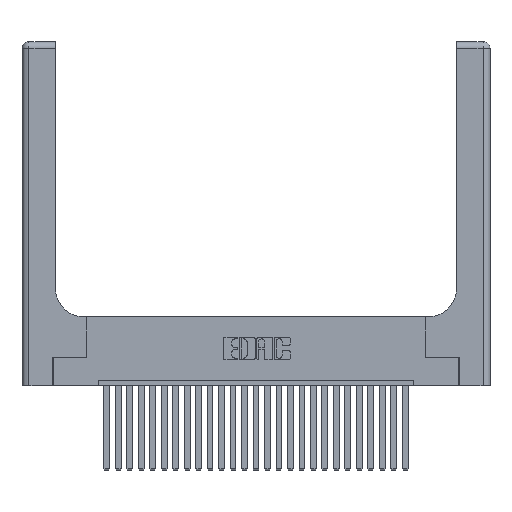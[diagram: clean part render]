
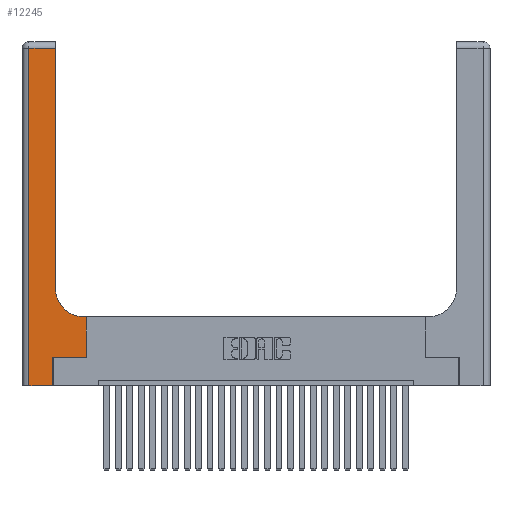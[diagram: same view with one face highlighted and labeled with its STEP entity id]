
A CAD part, top view. The second image highlights one B-rep face of the part: STEP entity #12245.
In plain terms, the highlighted planar face has unit normal (0, 0, 1).
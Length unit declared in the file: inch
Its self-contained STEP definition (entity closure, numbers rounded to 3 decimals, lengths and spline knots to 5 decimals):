
#540 = CARTESIAN_POINT ( 'NONE',  ( 0., 2.94, 0.37 ) ) ;
#699 = LINE ( 'NONE', #5644, #4050 ) ;
#837 = DIRECTION ( 'NONE',  ( 1., 0., 0. ) ) ;
#869 = PLANE ( 'NONE',  #12640 ) ;
#1617 = LINE ( 'NONE', #21561, #12179 ) ;
#1692 = VERTEX_POINT ( 'NONE', #2813 ) ;
#1924 = EDGE_CURVE ( 'NONE', #6714, #13691, #11876, .T. ) ;
#2122 = ORIENTED_EDGE ( 'NONE', *, *, #11858, .T. ) ;
#2713 = CARTESIAN_POINT ( 'NONE',  ( 0.5415, 0.85, 0.37 ) ) ;
#2813 = CARTESIAN_POINT ( 'NONE',  ( 0.5415, 0.6, 0.37 ) ) ;
#2981 = CARTESIAN_POINT ( 'NONE',  ( 0.5585, 0.25, 0.37 ) ) ;
#3144 = DIRECTION ( 'NONE',  ( 1., 0., 0. ) ) ;
#3164 = EDGE_LOOP ( 'NONE', ( #12885, #2122, #11545, #16739, #26783, #16769, #15127, #9532, #18774 ) ) ;
#3303 = VERTEX_POINT ( 'NONE', #8181 ) ;
#4050 = VECTOR ( 'NONE', #18064, 39.37008 ) ;
#4076 = VECTOR ( 'NONE', #3144, 39.37008 ) ;
#4863 = DIRECTION ( 'NONE',  ( 0., 0., -1. ) ) ;
#5048 = AXIS2_PLACEMENT_3D ( 'NONE', #2713, #23773, #837 ) ;
#5087 = DIRECTION ( 'NONE',  ( 0., -1., 0. ) ) ;
#5537 = VECTOR ( 'NONE', #9168, 39.37008 ) ;
#5644 = CARTESIAN_POINT ( 'NONE',  ( 0.2915, 3., 0.37 ) ) ;
#6230 = VERTEX_POINT ( 'NONE', #21611 ) ;
#6290 = VERTEX_POINT ( 'NONE', #13721 ) ;
#6550 = LINE ( 'NONE', #11457, #16449 ) ;
#6714 = VERTEX_POINT ( 'NONE', #19120 ) ;
#7165 = CARTESIAN_POINT ( 'NONE',  ( 0.2915, 0.85, 0.37 ) ) ;
#8181 = CARTESIAN_POINT ( 'NONE',  ( 0.269, 0., 0.37 ) ) ;
#8261 = EDGE_CURVE ( 'NONE', #3303, #6714, #21911, .T. ) ;
#8608 = CARTESIAN_POINT ( 'NONE',  ( 0.5585, 0.25, 0.37 ) ) ;
#9168 = DIRECTION ( 'NONE',  ( -1., 0., 0. ) ) ;
#9331 = LINE ( 'NONE', #8608, #20187 ) ;
#9532 = ORIENTED_EDGE ( 'NONE', *, *, #10983, .T. ) ;
#10983 = EDGE_CURVE ( 'NONE', #21089, #1692, #1617, .T. ) ;
#11071 = VERTEX_POINT ( 'NONE', #7165 ) ;
#11180 = CARTESIAN_POINT ( 'NONE',  ( 0.269, 0., 0.37 ) ) ;
#11457 = CARTESIAN_POINT ( 'NONE',  ( 0.06, 3., 0.37 ) ) ;
#11545 = ORIENTED_EDGE ( 'NONE', *, *, #21693, .T. ) ;
#11552 = VECTOR ( 'NONE', #15865, 39.37008 ) ;
#11620 = CARTESIAN_POINT ( 'NONE',  ( 0.269, 0.25, 0.37 ) ) ;
#11858 = EDGE_CURVE ( 'NONE', #6230, #6290, #14743, .T. ) ;
#11876 = LINE ( 'NONE', #11620, #11552 ) ;
#12179 = VECTOR ( 'NONE', #21657, 39.37008 ) ;
#12245 = ADVANCED_FACE ( 'NONE', ( #16404 ), #869, .F. ) ;
#12640 = AXIS2_PLACEMENT_3D ( 'NONE', #17492, #4863, #19596 ) ;
#12885 = ORIENTED_EDGE ( 'NONE', *, *, #14550, .T. ) ;
#13205 = EDGE_CURVE ( 'NONE', #21692, #3303, #23842, .T. ) ;
#13266 = DIRECTION ( 'NONE',  ( 0., 1., 0. ) ) ;
#13691 = VERTEX_POINT ( 'NONE', #2981 ) ;
#13721 = CARTESIAN_POINT ( 'NONE',  ( 0.06, 2.94, 0.37 ) ) ;
#14210 = EDGE_CURVE ( 'NONE', #13691, #21089, #9331, .T. ) ;
#14550 = EDGE_CURVE ( 'NONE', #11071, #6230, #699, .T. ) ;
#14743 = LINE ( 'NONE', #540, #5537 ) ;
#15127 = ORIENTED_EDGE ( 'NONE', *, *, #14210, .T. ) ;
#15865 = DIRECTION ( 'NONE',  ( 1., 0., 0. ) ) ;
#16029 = VECTOR ( 'NONE', #13266, 39.37008 ) ;
#16404 = FACE_OUTER_BOUND ( 'NONE', #3164, .T. ) ;
#16449 = VECTOR ( 'NONE', #5087, 39.37008 ) ;
#16739 = ORIENTED_EDGE ( 'NONE', *, *, #13205, .T. ) ;
#16769 = ORIENTED_EDGE ( 'NONE', *, *, #1924, .T. ) ;
#17492 = CARTESIAN_POINT ( 'NONE',  ( 0., 3., 0.37 ) ) ;
#17527 = CARTESIAN_POINT ( 'NONE',  ( 0.06, 0., 0.37 ) ) ;
#18064 = DIRECTION ( 'NONE',  ( 0., 1., 0. ) ) ;
#18774 = ORIENTED_EDGE ( 'NONE', *, *, #23929, .T. ) ;
#19120 = CARTESIAN_POINT ( 'NONE',  ( 0.269, 0.25, 0.37 ) ) ;
#19596 = DIRECTION ( 'NONE',  ( -1., 0., 0. ) ) ;
#20187 = VECTOR ( 'NONE', #25413, 39.37008 ) ;
#21089 = VERTEX_POINT ( 'NONE', #22232 ) ;
#21561 = CARTESIAN_POINT ( 'NONE',  ( 0.2915, 0.6, 0.37 ) ) ;
#21611 = CARTESIAN_POINT ( 'NONE',  ( 0.2915, 2.94, 0.37 ) ) ;
#21657 = DIRECTION ( 'NONE',  ( -1., 0., 0. ) ) ;
#21692 = VERTEX_POINT ( 'NONE', #17527 ) ;
#21693 = EDGE_CURVE ( 'NONE', #6290, #21692, #6550, .T. ) ;
#21911 = LINE ( 'NONE', #11180, #16029 ) ;
#22232 = CARTESIAN_POINT ( 'NONE',  ( 0.5585, 0.6, 0.37 ) ) ;
#23773 = DIRECTION ( 'NONE',  ( 0., 0., -1. ) ) ;
#23842 = LINE ( 'NONE', #25575, #4076 ) ;
#23929 = EDGE_CURVE ( 'NONE', #1692, #11071, #27228, .T. ) ;
#25413 = DIRECTION ( 'NONE',  ( 0., 1., 0. ) ) ;
#25575 = CARTESIAN_POINT ( 'NONE',  ( 0., 0., 0.37 ) ) ;
#26783 = ORIENTED_EDGE ( 'NONE', *, *, #8261, .T. ) ;
#27228 = CIRCLE ( 'NONE', #5048, 0.25 ) ;
